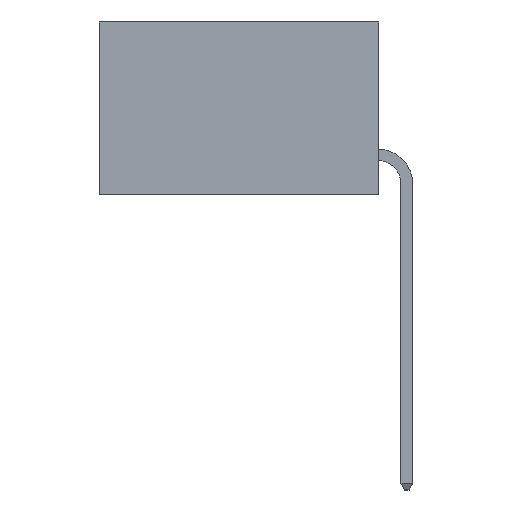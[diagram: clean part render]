
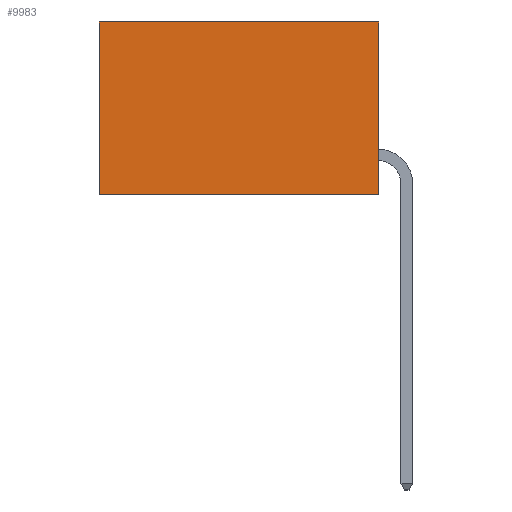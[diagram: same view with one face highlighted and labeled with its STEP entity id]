
A CAD part, left-side view. The second image highlights one B-rep face of the part: STEP entity #9983.
In plain terms, the highlighted planar face has unit normal (-1, 0, 0).
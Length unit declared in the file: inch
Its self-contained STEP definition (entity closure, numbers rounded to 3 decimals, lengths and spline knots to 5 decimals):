
#94 = ORIENTED_EDGE ( 'NONE', *, *, #9525, .T. ) ;
#830 = CARTESIAN_POINT ( 'NONE',  ( 0.2615, 0., -0.37 ) ) ;
#842 = DIRECTION ( 'NONE',  ( 1., 0., 0. ) ) ;
#1169 = CARTESIAN_POINT ( 'NONE',  ( 0.2615, 0., 0. ) ) ;
#1581 = ORIENTED_EDGE ( 'NONE', *, *, #11454, .F. ) ;
#1624 = FACE_OUTER_BOUND ( 'NONE', #2552, .T. ) ;
#1997 = AXIS2_PLACEMENT_3D ( 'NONE', #7339, #842, #7375 ) ;
#2552 = EDGE_LOOP ( 'NONE', ( #94, #8118, #1581, #7696 ) ) ;
#2832 = CARTESIAN_POINT ( 'NONE',  ( 0.2615, 0., -0.37 ) ) ;
#3092 = CARTESIAN_POINT ( 'NONE',  ( 0.2615, 0.6, -0.37 ) ) ;
#4433 = CARTESIAN_POINT ( 'NONE',  ( 0.2615, 0., 0. ) ) ;
#4700 = DIRECTION ( 'NONE',  ( 0., 0., -1. ) ) ;
#4712 = VECTOR ( 'NONE', #4700, 39.37008 ) ;
#4936 = CARTESIAN_POINT ( 'NONE',  ( 0.2615, 0.6, -0.37 ) ) ;
#4947 = VERTEX_POINT ( 'NONE', #5521 ) ;
#5521 = CARTESIAN_POINT ( 'NONE',  ( 0.2615, 0.6, 0. ) ) ;
#5525 = VECTOR ( 'NONE', #9493, 39.37008 ) ;
#5927 = DIRECTION ( 'NONE',  ( 0., 1., 0. ) ) ;
#6290 = EDGE_CURVE ( 'NONE', #9380, #8899, #7840, .T. ) ;
#6604 = VECTOR ( 'NONE', #5927, 39.37008 ) ;
#6714 = VECTOR ( 'NONE', #8444, 39.37008 ) ;
#7339 = CARTESIAN_POINT ( 'NONE',  ( 0.2615, 0., -0.37 ) ) ;
#7375 = DIRECTION ( 'NONE',  ( 0., 0., -1. ) ) ;
#7696 = ORIENTED_EDGE ( 'NONE', *, *, #8952, .T. ) ;
#7840 = LINE ( 'NONE', #9616, #5525 ) ;
#8118 = ORIENTED_EDGE ( 'NONE', *, *, #6290, .F. ) ;
#8444 = DIRECTION ( 'NONE',  ( 0., 0., -1. ) ) ;
#8899 = VERTEX_POINT ( 'NONE', #4936 ) ;
#8952 = EDGE_CURVE ( 'NONE', #9175, #4947, #11259, .T. ) ;
#9175 = VERTEX_POINT ( 'NONE', #4433 ) ;
#9380 = VERTEX_POINT ( 'NONE', #2832 ) ;
#9479 = LINE ( 'NONE', #3092, #6714 ) ;
#9493 = DIRECTION ( 'NONE',  ( 0., 1., 0. ) ) ;
#9525 = EDGE_CURVE ( 'NONE', #4947, #8899, #9479, .T. ) ;
#9616 = CARTESIAN_POINT ( 'NONE',  ( 0.2615, 0., -0.37 ) ) ;
#9838 = PLANE ( 'NONE',  #1997 ) ;
#9983 = ADVANCED_FACE ( 'NONE', ( #1624 ), #9838, .F. ) ;
#11259 = LINE ( 'NONE', #1169, #6604 ) ;
#11442 = LINE ( 'NONE', #830, #4712 ) ;
#11454 = EDGE_CURVE ( 'NONE', #9175, #9380, #11442, .T. ) ;
